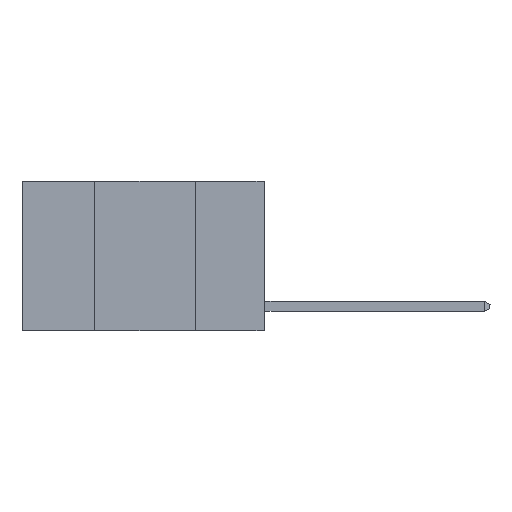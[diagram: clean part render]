
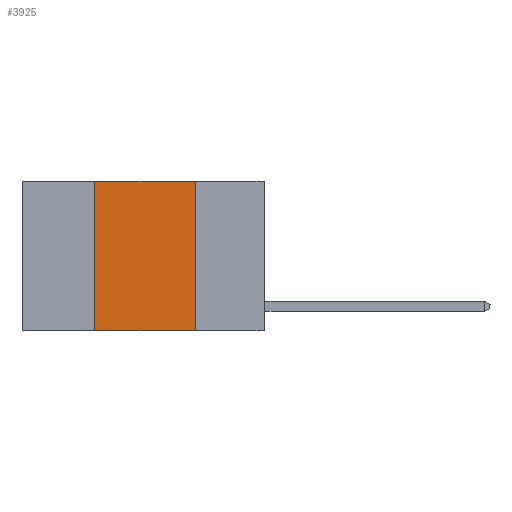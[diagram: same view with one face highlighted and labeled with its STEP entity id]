
A CAD part, left-side view. The second image highlights one B-rep face of the part: STEP entity #3925.
In plain terms, the highlighted planar face has unit normal (-1, 0, 0).
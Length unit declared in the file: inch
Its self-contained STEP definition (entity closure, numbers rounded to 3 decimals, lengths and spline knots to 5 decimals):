
#356 = CARTESIAN_POINT ( 'NONE',  ( 0., 0.42, 0. ) ) ;
#1303 = VECTOR ( 'NONE', #20301, 39.37008 ) ;
#1560 = ORIENTED_EDGE ( 'NONE', *, *, #8464, .F. ) ;
#2804 = PLANE ( 'NONE',  #6469 ) ;
#2912 = ORIENTED_EDGE ( 'NONE', *, *, #5960, .F. ) ;
#2958 = VECTOR ( 'NONE', #10171, 39.37008 ) ;
#3211 = ORIENTED_EDGE ( 'NONE', *, *, #22632, .T. ) ;
#3573 = VERTEX_POINT ( 'NONE', #20240 ) ;
#3639 = DIRECTION ( 'NONE',  ( 0., -1., 0. ) ) ;
#3797 = FACE_OUTER_BOUND ( 'NONE', #15411, .T. ) ;
#3867 = VECTOR ( 'NONE', #3639, 39.37008 ) ;
#3925 = ADVANCED_FACE ( 'NONE', ( #3797 ), #2804, .F. ) ;
#4440 = LINE ( 'NONE', #10914, #3867 ) ;
#4673 = CARTESIAN_POINT ( 'NONE',  ( 0., 0.6, -0.37 ) ) ;
#5960 = EDGE_CURVE ( 'NONE', #3573, #18127, #21729, .T. ) ;
#6070 = VERTEX_POINT ( 'NONE', #10999 ) ;
#6469 = AXIS2_PLACEMENT_3D ( 'NONE', #15657, #17467, #6532 ) ;
#6532 = DIRECTION ( 'NONE',  ( 0., 0., -1. ) ) ;
#6563 = VECTOR ( 'NONE', #14390, 39.37008 ) ;
#6853 = LINE ( 'NONE', #18426, #1303 ) ;
#8464 = EDGE_CURVE ( 'NONE', #18127, #19672, #4440, .T. ) ;
#10171 = DIRECTION ( 'NONE',  ( 0., -1., 0. ) ) ;
#10914 = CARTESIAN_POINT ( 'NONE',  ( 0., 0.6, 0. ) ) ;
#10999 = CARTESIAN_POINT ( 'NONE',  ( 0., 0.17, -0.37 ) ) ;
#13840 = CARTESIAN_POINT ( 'NONE',  ( 0., 0.17, 0. ) ) ;
#14390 = DIRECTION ( 'NONE',  ( 0., 0., 1. ) ) ;
#15411 = EDGE_LOOP ( 'NONE', ( #19364, #1560, #2912, #3211 ) ) ;
#15657 = CARTESIAN_POINT ( 'NONE',  ( 0., 0.6, 0. ) ) ;
#16846 = EDGE_CURVE ( 'NONE', #19672, #6070, #6853, .T. ) ;
#17467 = DIRECTION ( 'NONE',  ( 1., 0., 0. ) ) ;
#18127 = VERTEX_POINT ( 'NONE', #356 ) ;
#18135 = LINE ( 'NONE', #4673, #2958 ) ;
#18426 = CARTESIAN_POINT ( 'NONE',  ( 0., 0.17, 0. ) ) ;
#19364 = ORIENTED_EDGE ( 'NONE', *, *, #16846, .F. ) ;
#19672 = VERTEX_POINT ( 'NONE', #13840 ) ;
#20240 = CARTESIAN_POINT ( 'NONE',  ( 0., 0.42, -0.37 ) ) ;
#20301 = DIRECTION ( 'NONE',  ( 0., 0., -1. ) ) ;
#21649 = CARTESIAN_POINT ( 'NONE',  ( 0., 0.42, 0. ) ) ;
#21729 = LINE ( 'NONE', #21649, #6563 ) ;
#22632 = EDGE_CURVE ( 'NONE', #3573, #6070, #18135, .T. ) ;
